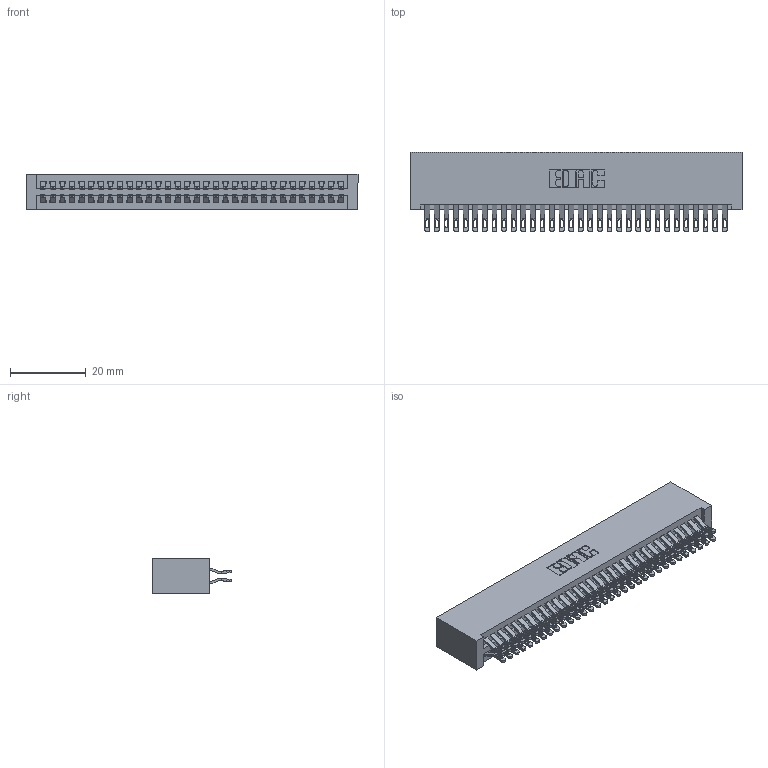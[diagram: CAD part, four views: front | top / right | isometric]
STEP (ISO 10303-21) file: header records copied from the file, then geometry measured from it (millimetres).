
FILE_DESCRIPTION (( 'STEP AP203' ), '1' );
FILE_NAME ('345-064-555-201.STEP', '2019-10-30T14:42:56', ( '' ), ( '' ), 'SwSTEP 2.0', 'SolidWorks 2016', '' );
FILE_SCHEMA (( 'CONFIG_CONTROL_DESIGN' ));
Length unit declared in the file: inch
Products named in the file (3): 345-292-001_555 Tail; 345 Part_No Mounting Lugs; 345-064-555-201
Assembly tree (65 placements, depth 2):
  345-064-555-201
    345 Part_No Mounting Lugs
    345-292-001_555 Tail  x64
Bounding box: 87.88 x 21.13 x 9.4 mm (x, y, z)
Volume: 9245.9 mm3; surface area: 14422.2 mm2
Topology: 65 solids, 65 shells, 3702 faces, 11645 edges, 7762 vertices
Faces by surface type: plane 2060, cylinder 1642
Entity records: 26503 total; most frequent: CARTESIAN_POINT 4486, ORIENTED_EDGE 4390, DIRECTION 3931, EDGE_CURVE 2195, VECTOR 1923, LINE 1923, VERTEX_POINT 1462, AXIS2_PLACEMENT_3D 1004
